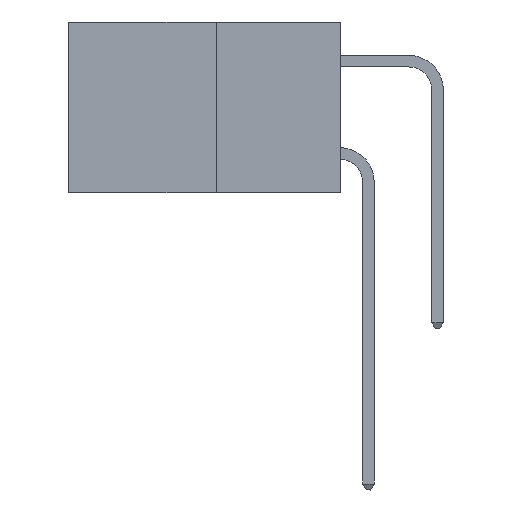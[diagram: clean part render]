
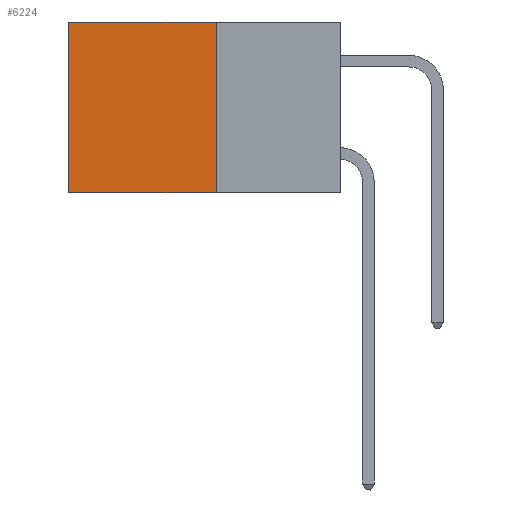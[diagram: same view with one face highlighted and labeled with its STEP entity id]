
A CAD part, left-side view. The second image highlights one B-rep face of the part: STEP entity #6224.
In plain terms, the highlighted planar face has unit normal (-1, 0, 0).
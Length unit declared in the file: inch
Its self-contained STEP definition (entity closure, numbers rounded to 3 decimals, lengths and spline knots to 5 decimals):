
#475 = CARTESIAN_POINT ( 'NONE',  ( 0.277, 0.27, -0.37 ) ) ;
#620 = ORIENTED_EDGE ( 'NONE', *, *, #4996, .F. ) ;
#869 = VECTOR ( 'NONE', #7534, 39.37008 ) ;
#966 = AXIS2_PLACEMENT_3D ( 'NONE', #7480, #11175, #3724 ) ;
#1615 = EDGE_CURVE ( 'NONE', #11035, #1731, #7550, .T. ) ;
#1642 = CARTESIAN_POINT ( 'NONE',  ( 0.277, 0.27, 0. ) ) ;
#1731 = VERTEX_POINT ( 'NONE', #2294 ) ;
#2294 = CARTESIAN_POINT ( 'NONE',  ( 0.277, 0.59, 0. ) ) ;
#2479 = PLANE ( 'NONE',  #966 ) ;
#3220 = VERTEX_POINT ( 'NONE', #12129 ) ;
#3724 = DIRECTION ( 'NONE',  ( 0., 0., -1. ) ) ;
#3860 = VECTOR ( 'NONE', #12989, 39.37008 ) ;
#4466 = CARTESIAN_POINT ( 'NONE',  ( 0.277, 0.27, 0. ) ) ;
#4671 = EDGE_CURVE ( 'NONE', #11035, #11132, #6664, .T. ) ;
#4902 = ORIENTED_EDGE ( 'NONE', *, *, #4671, .F. ) ;
#4996 = EDGE_CURVE ( 'NONE', #11132, #3220, #11837, .T. ) ;
#5883 = EDGE_CURVE ( 'NONE', #1731, #3220, #13702, .T. ) ;
#6224 = ADVANCED_FACE ( 'NONE', ( #12970 ), #2479, .F. ) ;
#6664 = LINE ( 'NONE', #14539, #12799 ) ;
#7008 = EDGE_LOOP ( 'NONE', ( #10287, #620, #4902, #11440 ) ) ;
#7480 = CARTESIAN_POINT ( 'NONE',  ( 0.277, 0.27, -0.37 ) ) ;
#7534 = DIRECTION ( 'NONE',  ( 0., 1., 0. ) ) ;
#7550 = LINE ( 'NONE', #4466, #869 ) ;
#8624 = VECTOR ( 'NONE', #11425, 39.37008 ) ;
#10195 = CARTESIAN_POINT ( 'NONE',  ( 0.277, 0.27, -0.37 ) ) ;
#10287 = ORIENTED_EDGE ( 'NONE', *, *, #5883, .T. ) ;
#11035 = VERTEX_POINT ( 'NONE', #1642 ) ;
#11132 = VERTEX_POINT ( 'NONE', #475 ) ;
#11175 = DIRECTION ( 'NONE',  ( 1., 0., 0. ) ) ;
#11425 = DIRECTION ( 'NONE',  ( 0., 1., 0. ) ) ;
#11440 = ORIENTED_EDGE ( 'NONE', *, *, #1615, .T. ) ;
#11774 = CARTESIAN_POINT ( 'NONE',  ( 0.277, 0.59, -0.37 ) ) ;
#11837 = LINE ( 'NONE', #10195, #8624 ) ;
#12129 = CARTESIAN_POINT ( 'NONE',  ( 0.277, 0.59, -0.37 ) ) ;
#12799 = VECTOR ( 'NONE', #13338, 39.37008 ) ;
#12970 = FACE_OUTER_BOUND ( 'NONE', #7008, .T. ) ;
#12989 = DIRECTION ( 'NONE',  ( 0., 0., -1. ) ) ;
#13338 = DIRECTION ( 'NONE',  ( 0., 0., -1. ) ) ;
#13702 = LINE ( 'NONE', #11774, #3860 ) ;
#14539 = CARTESIAN_POINT ( 'NONE',  ( 0.277, 0.27, -0.37 ) ) ;
